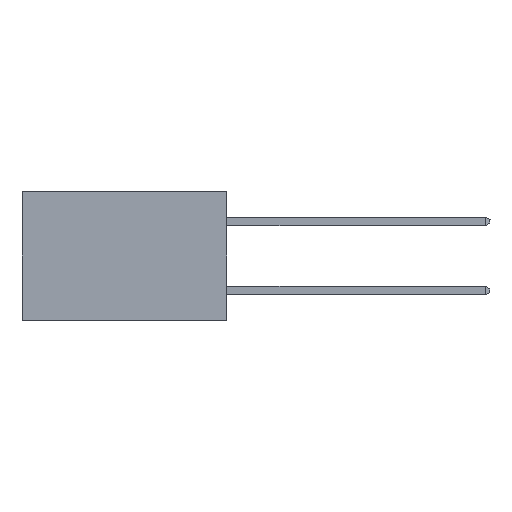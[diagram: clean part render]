
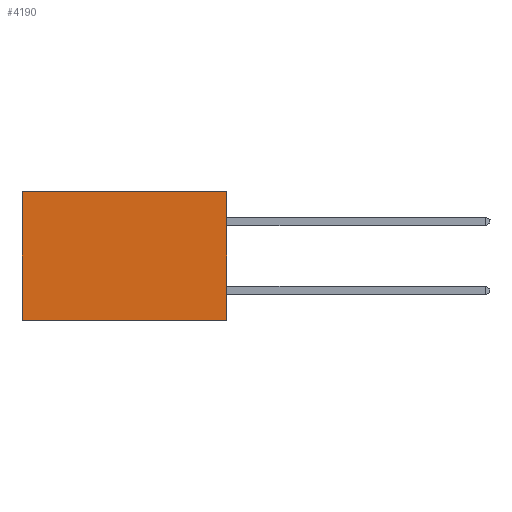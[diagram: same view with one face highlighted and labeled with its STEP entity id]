
A CAD part, left-side view. The second image highlights one B-rep face of the part: STEP entity #4190.
In plain terms, the highlighted planar face has unit normal (-1, 0, 0).
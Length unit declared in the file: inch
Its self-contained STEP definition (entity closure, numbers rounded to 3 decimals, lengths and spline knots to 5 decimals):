
#230 = CARTESIAN_POINT ( 'NONE',  ( 0.277, 0., -0.37 ) ) ;
#261 = CARTESIAN_POINT ( 'NONE',  ( 0.277, 0., -0.37 ) ) ;
#292 = DIRECTION ( 'NONE',  ( 0., 1., 0. ) ) ;
#298 = VERTEX_POINT ( 'NONE', #5094 ) ;
#479 = AXIS2_PLACEMENT_3D ( 'NONE', #1997, #4663, #8358 ) ;
#556 = VECTOR ( 'NONE', #292, 39.37008 ) ;
#848 = VERTEX_POINT ( 'NONE', #6537 ) ;
#903 = EDGE_CURVE ( 'NONE', #2698, #1056, #1405, .T. ) ;
#931 = DIRECTION ( 'NONE',  ( 0., 1., 0. ) ) ;
#1032 = CARTESIAN_POINT ( 'NONE',  ( 0.277, 0., 0. ) ) ;
#1056 = VERTEX_POINT ( 'NONE', #5255 ) ;
#1405 = LINE ( 'NONE', #261, #7898 ) ;
#1639 = ORIENTED_EDGE ( 'NONE', *, *, #3401, .T. ) ;
#1778 = ORIENTED_EDGE ( 'NONE', *, *, #6803, .F. ) ;
#1997 = CARTESIAN_POINT ( 'NONE',  ( 0.277, 0., -0.37 ) ) ;
#2031 = ORIENTED_EDGE ( 'NONE', *, *, #903, .F. ) ;
#2044 = PLANE ( 'NONE',  #479 ) ;
#2126 = FACE_OUTER_BOUND ( 'NONE', #4106, .T. ) ;
#2698 = VERTEX_POINT ( 'NONE', #5618 ) ;
#3401 = EDGE_CURVE ( 'NONE', #2698, #298, #4142, .T. ) ;
#4106 = EDGE_LOOP ( 'NONE', ( #8139, #1778, #2031, #1639 ) ) ;
#4142 = LINE ( 'NONE', #1032, #556 ) ;
#4190 = ADVANCED_FACE ( 'NONE', ( #2126 ), #2044, .F. ) ;
#4473 = DIRECTION ( 'NONE',  ( 0., 0., -1. ) ) ;
#4501 = CARTESIAN_POINT ( 'NONE',  ( 0.277, 0.59, -0.37 ) ) ;
#4621 = EDGE_CURVE ( 'NONE', #298, #848, #7842, .T. ) ;
#4663 = DIRECTION ( 'NONE',  ( 1., 0., 0. ) ) ;
#5094 = CARTESIAN_POINT ( 'NONE',  ( 0.277, 0.59, 0. ) ) ;
#5255 = CARTESIAN_POINT ( 'NONE',  ( 0.277, 0., -0.37 ) ) ;
#5618 = CARTESIAN_POINT ( 'NONE',  ( 0.277, 0., 0. ) ) ;
#5999 = LINE ( 'NONE', #230, #7410 ) ;
#6443 = DIRECTION ( 'NONE',  ( 0., 0., -1. ) ) ;
#6488 = VECTOR ( 'NONE', #4473, 39.37008 ) ;
#6537 = CARTESIAN_POINT ( 'NONE',  ( 0.277, 0.59, -0.37 ) ) ;
#6803 = EDGE_CURVE ( 'NONE', #1056, #848, #5999, .T. ) ;
#7410 = VECTOR ( 'NONE', #931, 39.37008 ) ;
#7842 = LINE ( 'NONE', #4501, #6488 ) ;
#7898 = VECTOR ( 'NONE', #6443, 39.37008 ) ;
#8139 = ORIENTED_EDGE ( 'NONE', *, *, #4621, .T. ) ;
#8358 = DIRECTION ( 'NONE',  ( 0., 0., -1. ) ) ;
